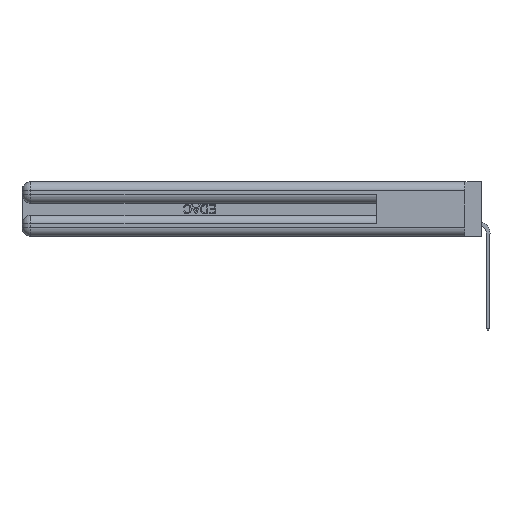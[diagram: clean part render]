
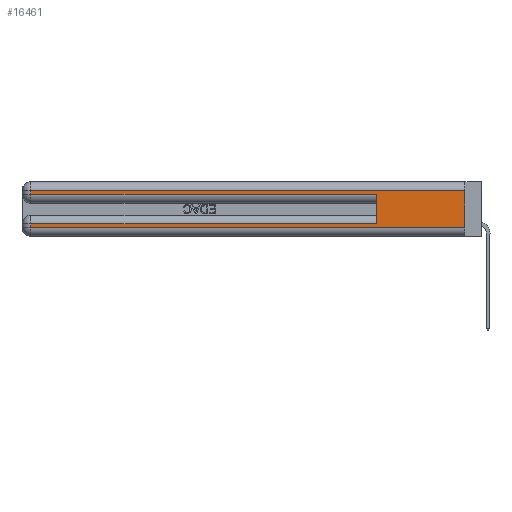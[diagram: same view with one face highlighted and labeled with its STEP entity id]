
A CAD part, left-side view. The second image highlights one B-rep face of the part: STEP entity #16461.
In plain terms, the highlighted planar face has unit normal (-1, 0, 0).
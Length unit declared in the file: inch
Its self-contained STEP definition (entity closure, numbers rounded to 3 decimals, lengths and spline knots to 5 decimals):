
#921 = CARTESIAN_POINT ( 'NONE',  ( 0., 2.94, 0.085 ) ) ;
#1224 = CARTESIAN_POINT ( 'NONE',  ( 0., 2.94, 0.37 ) ) ;
#1490 = ORIENTED_EDGE ( 'NONE', *, *, #21760, .T. ) ;
#1997 = LINE ( 'NONE', #34654, #38603 ) ;
#2790 = DIRECTION ( 'NONE',  ( 0., 1., 0. ) ) ;
#3353 = CARTESIAN_POINT ( 'NONE',  ( 0., 0., 0.37 ) ) ;
#3736 = ORIENTED_EDGE ( 'NONE', *, *, #21483, .F. ) ;
#3759 = ORIENTED_EDGE ( 'NONE', *, *, #7000, .T. ) ;
#3961 = CARTESIAN_POINT ( 'NONE',  ( 0., 2.94, 0.37 ) ) ;
#4140 = EDGE_CURVE ( 'NONE', #32815, #22465, #1997, .T. ) ;
#4719 = EDGE_LOOP ( 'NONE', ( #3736, #1490, #35950, #36668, #34334, #3759, #17827, #22398 ) ) ;
#5455 = VECTOR ( 'NONE', #9665, 39.37008 ) ;
#5685 = EDGE_CURVE ( 'NONE', #37919, #23333, #35662, .T. ) ;
#6082 = VERTEX_POINT ( 'NONE', #33898 ) ;
#6414 = EDGE_CURVE ( 'NONE', #33393, #15331, #16870, .T. ) ;
#7000 = EDGE_CURVE ( 'NONE', #32815, #37919, #28604, .T. ) ;
#7070 = EDGE_CURVE ( 'NONE', #15331, #22465, #27625, .T. ) ;
#7310 = DIRECTION ( 'NONE',  ( 1., 0., 0. ) ) ;
#8555 = DIRECTION ( 'NONE',  ( 0., -1., 0. ) ) ;
#9105 = VERTEX_POINT ( 'NONE', #26695 ) ;
#9665 = DIRECTION ( 'NONE',  ( 0., -1., 0. ) ) ;
#9861 = DIRECTION ( 'NONE',  ( 0., 0., -1. ) ) ;
#12308 = CARTESIAN_POINT ( 'NONE',  ( 0., 0., 0.085 ) ) ;
#13296 = DIRECTION ( 'NONE',  ( 0., 1., 0. ) ) ;
#13479 = DIRECTION ( 'NONE',  ( 0., 0., -1. ) ) ;
#15331 = VERTEX_POINT ( 'NONE', #20946 ) ;
#15948 = DIRECTION ( 'NONE',  ( 0., 0., -1. ) ) ;
#16461 = ADVANCED_FACE ( 'NONE', ( #35873 ), #16798, .F. ) ;
#16798 = PLANE ( 'NONE',  #30116 ) ;
#16870 = LINE ( 'NONE', #1224, #31847 ) ;
#17827 = ORIENTED_EDGE ( 'NONE', *, *, #5685, .T. ) ;
#18170 = CARTESIAN_POINT ( 'NONE',  ( 0., 0., 0.285 ) ) ;
#19726 = VECTOR ( 'NONE', #24958, 39.37008 ) ;
#20946 = CARTESIAN_POINT ( 'NONE',  ( 0., 2.94, 0.285 ) ) ;
#21483 = EDGE_CURVE ( 'NONE', #6082, #9105, #25650, .T. ) ;
#21760 = EDGE_CURVE ( 'NONE', #6082, #33393, #28457, .T. ) ;
#22398 = ORIENTED_EDGE ( 'NONE', *, *, #32490, .T. ) ;
#22465 = VERTEX_POINT ( 'NONE', #28366 ) ;
#23333 = VERTEX_POINT ( 'NONE', #23562 ) ;
#23562 = CARTESIAN_POINT ( 'NONE',  ( 0., 2.94, 0.06 ) ) ;
#24639 = CARTESIAN_POINT ( 'NONE',  ( 0., 0., 0.06 ) ) ;
#24648 = VECTOR ( 'NONE', #13296, 39.37008 ) ;
#24958 = DIRECTION ( 'NONE',  ( 0., 0., -1. ) ) ;
#25650 = LINE ( 'NONE', #3353, #27966 ) ;
#26695 = CARTESIAN_POINT ( 'NONE',  ( 0., 0., 0.06 ) ) ;
#27140 = VECTOR ( 'NONE', #8555, 39.37008 ) ;
#27625 = LINE ( 'NONE', #18170, #27140 ) ;
#27966 = VECTOR ( 'NONE', #9861, 39.37008 ) ;
#28366 = CARTESIAN_POINT ( 'NONE',  ( 0., 0.6, 0.285 ) ) ;
#28457 = LINE ( 'NONE', #31153, #24648 ) ;
#28604 = LINE ( 'NONE', #12308, #35133 ) ;
#30116 = AXIS2_PLACEMENT_3D ( 'NONE', #34605, #7310, #13479 ) ;
#30363 = LINE ( 'NONE', #24639, #5455 ) ;
#31153 = CARTESIAN_POINT ( 'NONE',  ( 0., 0., 0.31 ) ) ;
#31847 = VECTOR ( 'NONE', #15948, 39.37008 ) ;
#32193 = CARTESIAN_POINT ( 'NONE',  ( 0., 2.94, 0.31 ) ) ;
#32490 = EDGE_CURVE ( 'NONE', #23333, #9105, #30363, .T. ) ;
#32815 = VERTEX_POINT ( 'NONE', #38512 ) ;
#33393 = VERTEX_POINT ( 'NONE', #32193 ) ;
#33898 = CARTESIAN_POINT ( 'NONE',  ( 0., 0., 0.31 ) ) ;
#34334 = ORIENTED_EDGE ( 'NONE', *, *, #4140, .F. ) ;
#34605 = CARTESIAN_POINT ( 'NONE',  ( 0., 0., 0.37 ) ) ;
#34654 = CARTESIAN_POINT ( 'NONE',  ( 0., 0.6, 0.145 ) ) ;
#35133 = VECTOR ( 'NONE', #2790, 39.37008 ) ;
#35662 = LINE ( 'NONE', #3961, #19726 ) ;
#35873 = FACE_OUTER_BOUND ( 'NONE', #4719, .T. ) ;
#35950 = ORIENTED_EDGE ( 'NONE', *, *, #6414, .T. ) ;
#36668 = ORIENTED_EDGE ( 'NONE', *, *, #7070, .T. ) ;
#37665 = DIRECTION ( 'NONE',  ( 0., 0., 1. ) ) ;
#37919 = VERTEX_POINT ( 'NONE', #921 ) ;
#38512 = CARTESIAN_POINT ( 'NONE',  ( 0., 0.6, 0.085 ) ) ;
#38603 = VECTOR ( 'NONE', #37665, 39.37008 ) ;
